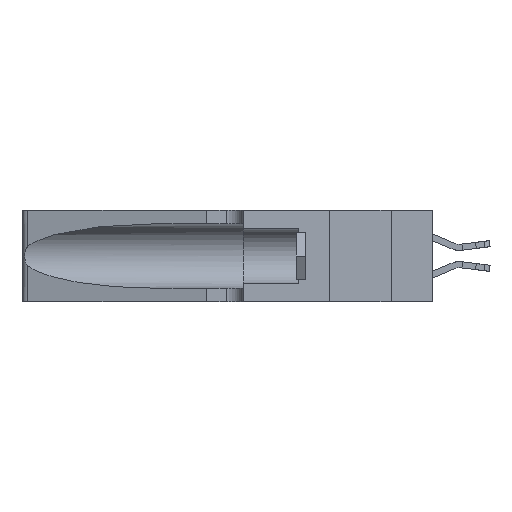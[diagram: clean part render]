
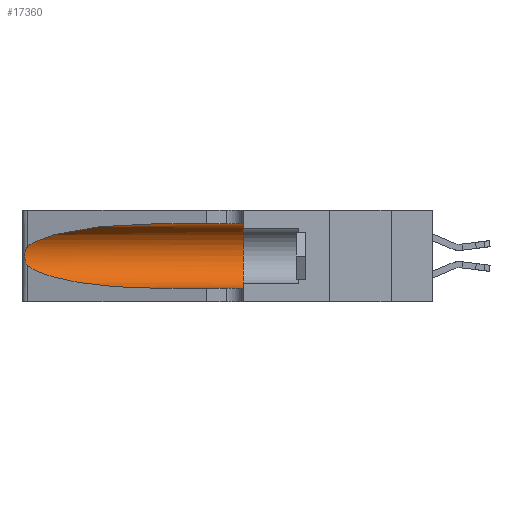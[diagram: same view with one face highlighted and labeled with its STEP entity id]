
A CAD part, left-side view. The second image highlights one B-rep face of the part: STEP entity #17360.
In plain terms, the highlighted cylindrical face has radius 3.308 mm (diameter 6.617 mm), a partial arc.
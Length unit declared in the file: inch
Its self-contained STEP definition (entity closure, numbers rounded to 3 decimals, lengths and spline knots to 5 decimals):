
#513 = DIRECTION ( 'NONE',  ( 0., -1., 0. ) ) ;
#611 = CIRCLE ( 'NONE', #8528, 0.13025 ) ;
#1071 = EDGE_CURVE ( 'NONE', #20834, #18336, #3442, .T. ) ;
#1416 = EDGE_CURVE ( 'NONE', #18336, #5673, #3306, .T. ) ;
#1963 = EDGE_CURVE ( 'NONE', #6054, #20834, #2736, .T. ) ;
#2189 = CARTESIAN_POINT ( 'NONE',  ( 0.1305, 0.72297, 0.05475 ) ) ;
#2246 = CARTESIAN_POINT ( 'NONE',  ( 0.25487, 1.22718, 0.22369 ) ) ;
#2707 = EDGE_LOOP ( 'NONE', ( #6223, #15154, #19994, #16538, #11610, #17476 ) ) ;
#2736 =( BOUNDED_CURVE ( )  B_SPLINE_CURVE ( 3, ( #7485, #7422, #14585, #2246 ),
 .UNSPECIFIED., .F., .F. ) 
 B_SPLINE_CURVE_WITH_KNOTS ( ( 4, 4 ),
 ( 1.5708, 2.84003 ),
 .UNSPECIFIED. ) 
 CURVE ( )  GEOMETRIC_REPRESENTATION_ITEM ( )  RATIONAL_B_SPLINE_CURVE ( ( 1., 0.87, 0.87, 1. ) ) 
 REPRESENTATION_ITEM ( '' )  );
#3306 =( BOUNDED_CURVE ( )  B_SPLINE_CURVE ( 3, ( #10558, #10262, #12213, #2189 ),
 .UNSPECIFIED., .F., .F. ) 
 B_SPLINE_CURVE_WITH_KNOTS ( ( 4, 4 ),
 ( 3.44316, 4.71239 ),
 .UNSPECIFIED. ) 
 CURVE ( )  GEOMETRIC_REPRESENTATION_ITEM ( )  RATIONAL_B_SPLINE_CURVE ( ( 1., 0.87, 0.87, 1. ) ) 
 REPRESENTATION_ITEM ( '' )  );
#3442 = B_SPLINE_CURVE_WITH_KNOTS ( 'NONE', 3,
 ( #10232, #16094, #16071, #16210, #16193, #16325, #16296, #16459, #16421, #16529, #16504, #16604, #16601, #16787 ),
 .UNSPECIFIED., .F., .F.,
 ( 4, 2, 2, 2, 2, 2, 4 ),
 ( 0., 0.00027, 0.00053, 0.00107, 0.0016, 0.00187, 0.00214 ),
 .UNSPECIFIED. ) ;
#3713 = VERTEX_POINT ( 'NONE', #11385 ) ;
#4424 = LINE ( 'NONE', #14383, #8608 ) ;
#5673 = VERTEX_POINT ( 'NONE', #16000 ) ;
#6054 = VERTEX_POINT ( 'NONE', #17216 ) ;
#6223 = ORIENTED_EDGE ( 'NONE', *, *, #1963, .T. ) ;
#6923 = CARTESIAN_POINT ( 'NONE',  ( 0.1305, 1.61858, 0.185 ) ) ;
#7119 = CARTESIAN_POINT ( 'NONE',  ( 0.1305, 1.61858, 0.05475 ) ) ;
#7335 = FACE_OUTER_BOUND ( 'NONE', #2707, .T. ) ;
#7349 = DIRECTION ( 'NONE',  ( 0., 1., 0. ) ) ;
#7422 = CARTESIAN_POINT ( 'NONE',  ( 0.18966, 0.96281, 0.31525 ) ) ;
#7485 = CARTESIAN_POINT ( 'NONE',  ( 0.1305, 0.72297, 0.31525 ) ) ;
#8528 = AXIS2_PLACEMENT_3D ( 'NONE', #17318, #7349, #18934 ) ;
#8608 = VECTOR ( 'NONE', #513, 39.37008 ) ;
#8668 = DIRECTION ( 'NONE',  ( 0., 0., -1. ) ) ;
#8786 = VECTOR ( 'NONE', #8855, 39.37008 ) ;
#8855 = DIRECTION ( 'NONE',  ( 0., -1., 0. ) ) ;
#10232 = CARTESIAN_POINT ( 'NONE',  ( 0.25487, 1.22718, 0.22369 ) ) ;
#10262 = CARTESIAN_POINT ( 'NONE',  ( 0.2373, 1.15595, 0.08982 ) ) ;
#10558 = CARTESIAN_POINT ( 'NONE',  ( 0.25487, 1.22718, 0.14631 ) ) ;
#11250 = CARTESIAN_POINT ( 'NONE',  ( 0.25487, 1.22718, 0.14631 ) ) ;
#11385 = CARTESIAN_POINT ( 'NONE',  ( 0.1305, 0.35, 0.05475 ) ) ;
#11610 = ORIENTED_EDGE ( 'NONE', *, *, #16371, .F. ) ;
#12132 = EDGE_CURVE ( 'NONE', #6054, #18537, #4424, .T. ) ;
#12213 = CARTESIAN_POINT ( 'NONE',  ( 0.18966, 0.96281, 0.05475 ) ) ;
#14383 = CARTESIAN_POINT ( 'NONE',  ( 0.1305, 1.61858, 0.31525 ) ) ;
#14585 = CARTESIAN_POINT ( 'NONE',  ( 0.2373, 1.15595, 0.28018 ) ) ;
#15154 = ORIENTED_EDGE ( 'NONE', *, *, #1071, .T. ) ;
#15365 = EDGE_CURVE ( 'NONE', #5673, #3713, #16554, .T. ) ;
#15664 = CYLINDRICAL_SURFACE ( 'NONE', #20500, 0.13025 ) ;
#16000 = CARTESIAN_POINT ( 'NONE',  ( 0.1305, 0.72297, 0.05475 ) ) ;
#16071 = CARTESIAN_POINT ( 'NONE',  ( 0.25639, 1.23184, 0.21858 ) ) ;
#16094 = CARTESIAN_POINT ( 'NONE',  ( 0.25555, 1.22994, 0.2215 ) ) ;
#16193 = CARTESIAN_POINT ( 'NONE',  ( 0.25854, 1.2359, 0.20912 ) ) ;
#16210 = CARTESIAN_POINT ( 'NONE',  ( 0.25787, 1.23484, 0.2124 ) ) ;
#16296 = CARTESIAN_POINT ( 'NONE',  ( 0.26075, 1.23896, 0.19203 ) ) ;
#16325 = CARTESIAN_POINT ( 'NONE',  ( 0.26018, 1.23835, 0.19895 ) ) ;
#16371 = EDGE_CURVE ( 'NONE', #18537, #3713, #611, .T. ) ;
#16421 = CARTESIAN_POINT ( 'NONE',  ( 0.26017, 1.23833, 0.17102 ) ) ;
#16459 = CARTESIAN_POINT ( 'NONE',  ( 0.26075, 1.23896, 0.178 ) ) ;
#16504 = CARTESIAN_POINT ( 'NONE',  ( 0.25789, 1.23486, 0.15765 ) ) ;
#16529 = CARTESIAN_POINT ( 'NONE',  ( 0.25856, 1.23593, 0.16098 ) ) ;
#16538 = ORIENTED_EDGE ( 'NONE', *, *, #15365, .T. ) ;
#16554 = LINE ( 'NONE', #7119, #8786 ) ;
#16601 = CARTESIAN_POINT ( 'NONE',  ( 0.25555, 1.22993, 0.14849 ) ) ;
#16604 = CARTESIAN_POINT ( 'NONE',  ( 0.25639, 1.23186, 0.15144 ) ) ;
#16787 = CARTESIAN_POINT ( 'NONE',  ( 0.25487, 1.22718, 0.14631 ) ) ;
#17216 = CARTESIAN_POINT ( 'NONE',  ( 0.1305, 0.72297, 0.31525 ) ) ;
#17318 = CARTESIAN_POINT ( 'NONE',  ( 0.1305, 0.35, 0.185 ) ) ;
#17360 = ADVANCED_FACE ( 'NONE', ( #7335 ), #15664, .F. ) ;
#17476 = ORIENTED_EDGE ( 'NONE', *, *, #12132, .F. ) ;
#18336 = VERTEX_POINT ( 'NONE', #11250 ) ;
#18536 = DIRECTION ( 'NONE',  ( 0., -1., 0. ) ) ;
#18537 = VERTEX_POINT ( 'NONE', #21437 ) ;
#18934 = DIRECTION ( 'NONE',  ( 0., 0., 1. ) ) ;
#19904 = CARTESIAN_POINT ( 'NONE',  ( 0.25487, 1.22718, 0.22369 ) ) ;
#19994 = ORIENTED_EDGE ( 'NONE', *, *, #1416, .T. ) ;
#20500 = AXIS2_PLACEMENT_3D ( 'NONE', #6923, #18536, #8668 ) ;
#20834 = VERTEX_POINT ( 'NONE', #19904 ) ;
#21437 = CARTESIAN_POINT ( 'NONE',  ( 0.1305, 0.35, 0.31525 ) ) ;
